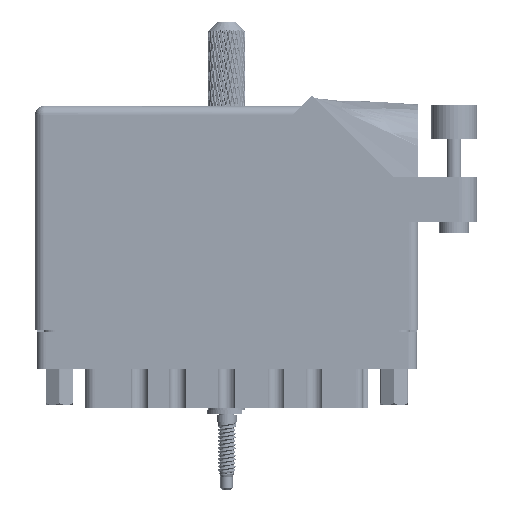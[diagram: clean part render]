
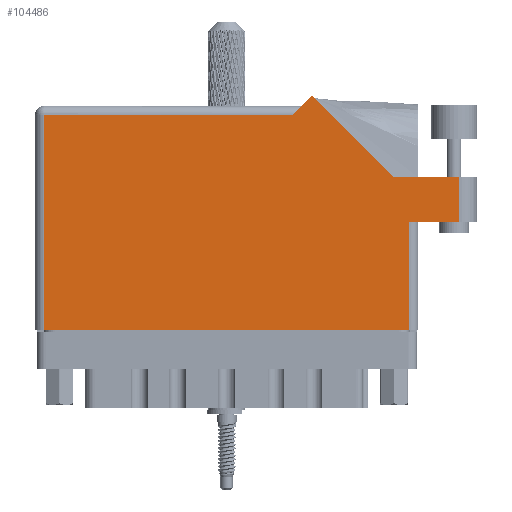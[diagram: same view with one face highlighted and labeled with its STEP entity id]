
A CAD part, front view. The second image highlights one B-rep face of the part: STEP entity #104486.
In plain terms, the highlighted face is planar.
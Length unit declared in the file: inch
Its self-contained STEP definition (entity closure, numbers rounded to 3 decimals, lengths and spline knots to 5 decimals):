
#1196 = LINE ( 'NONE', #117034, #110915 ) ;
#1963 = CARTESIAN_POINT ( 'NONE',  ( 2.55, 0., 0. ) ) ;
#3700 = VERTEX_POINT ( 'NONE', #48009 ) ;
#4929 = CARTESIAN_POINT ( 'NONE',  ( 3.012, 1.044, 0. ) ) ;
#5203 = EDGE_CURVE ( 'NONE', #57094, #62060, #86140, .T. ) ;
#5409 = EDGE_CURVE ( 'NONE', #79869, #85495, #1196, .T. ) ;
#7006 = ORIENTED_EDGE ( 'NONE', *, *, #32670, .T. ) ;
#7278 = DIRECTION ( 'NONE',  ( 0., 0., -1. ) ) ;
#7817 = VERTEX_POINT ( 'NONE', #110042 ) ;
#8028 = CARTESIAN_POINT ( 'NONE',  ( 0.062, 0., 0. ) ) ;
#8616 = VERTEX_POINT ( 'NONE', #47027 ) ;
#12531 = DIRECTION ( 'NONE',  ( -1., 0., 0. ) ) ;
#17126 = DIRECTION ( 'NONE',  ( 0., -1., 0. ) ) ;
#17730 = AXIS2_PLACEMENT_3D ( 'NONE', #115320, #7278, #95052 ) ;
#18593 = DIRECTION ( 'NONE',  ( 1., 0., 0. ) ) ;
#18639 = ORIENTED_EDGE ( 'NONE', *, *, #60508, .T. ) ;
#21123 = ORIENTED_EDGE ( 'NONE', *, *, #5409, .T. ) ;
#22456 = ORIENTED_EDGE ( 'NONE', *, *, #83307, .T. ) ;
#23489 = EDGE_CURVE ( 'NONE', #85495, #8616, #124495, .T. ) ;
#26390 = VECTOR ( 'NONE', #115205, 39.37008 ) ;
#27589 = CARTESIAN_POINT ( 'NONE',  ( 1.757, 1.468, 0. ) ) ;
#28414 = DIRECTION ( 'NONE',  ( -0.707, 0.707, 0. ) ) ;
#29213 = VERTEX_POINT ( 'NONE', #86836 ) ;
#31591 = VECTOR ( 'NONE', #28414, 39.37008 ) ;
#32055 = CARTESIAN_POINT ( 'NONE',  ( 2.887, 1.044, 0. ) ) ;
#32670 = EDGE_CURVE ( 'NONE', #8616, #7817, #53519, .T. ) ;
#35120 = ORIENTED_EDGE ( 'NONE', *, *, #47902, .T. ) ;
#39615 = DIRECTION ( 'NONE',  ( -0.707, -0.707, 0. ) ) ;
#47027 = CARTESIAN_POINT ( 'NONE',  ( 2.887, 0.737, 0. ) ) ;
#47902 = EDGE_CURVE ( 'NONE', #3700, #57094, #87890, .T. ) ;
#48009 = CARTESIAN_POINT ( 'NONE',  ( 1.88971, 1.60071, 0. ) ) ;
#48913 = CARTESIAN_POINT ( 'NONE',  ( 0., 1.468, 0. ) ) ;
#50754 = VECTOR ( 'NONE', #39615, 39.37008 ) ;
#50826 = ORIENTED_EDGE ( 'NONE', *, *, #23489, .T. ) ;
#53226 = EDGE_LOOP ( 'NONE', ( #50826, #7006, #22456, #83543, #35120, #107924, #18639, #68264, #21123 ) ) ;
#53519 = LINE ( 'NONE', #32055, #107724 ) ;
#57094 = VERTEX_POINT ( 'NONE', #27589 ) ;
#57649 = CARTESIAN_POINT ( 'NONE',  ( 2.44642, 1.044, 0. ) ) ;
#60508 = EDGE_CURVE ( 'NONE', #62060, #29213, #88337, .T. ) ;
#62060 = VERTEX_POINT ( 'NONE', #64249 ) ;
#62989 = DIRECTION ( 'NONE',  ( 0., 1., 0. ) ) ;
#64249 = CARTESIAN_POINT ( 'NONE',  ( 0.062, 1.468, 0. ) ) ;
#64496 = CARTESIAN_POINT ( 'NONE',  ( 2.55, 0.737, 0. ) ) ;
#68237 = CARTESIAN_POINT ( 'NONE',  ( 2.612, 0.737, 0. ) ) ;
#68264 = ORIENTED_EDGE ( 'NONE', *, *, #73088, .T. ) ;
#73088 = EDGE_CURVE ( 'NONE', #29213, #79869, #78944, .T. ) ;
#73712 = VECTOR ( 'NONE', #12531, 39.37008 ) ;
#78944 = LINE ( 'NONE', #107006, #26390 ) ;
#79869 = VERTEX_POINT ( 'NONE', #1963 ) ;
#83307 = EDGE_CURVE ( 'NONE', #7817, #120252, #83530, .T. ) ;
#83530 = LINE ( 'NONE', #4929, #126783 ) ;
#83543 = ORIENTED_EDGE ( 'NONE', *, *, #114080, .T. ) ;
#85495 = VERTEX_POINT ( 'NONE', #64496 ) ;
#86140 = LINE ( 'NONE', #48913, #73712 ) ;
#86810 = DIRECTION ( 'NONE',  ( 0., 1., 0. ) ) ;
#86836 = CARTESIAN_POINT ( 'NONE',  ( 0.062, 0., 0. ) ) ;
#87890 = LINE ( 'NONE', #88465, #50754 ) ;
#88337 = LINE ( 'NONE', #8028, #100730 ) ;
#88465 = CARTESIAN_POINT ( 'NONE',  ( 1.819, 1.53, 0. ) ) ;
#95052 = DIRECTION ( 'NONE',  ( -1., 0., 0. ) ) ;
#96975 = FACE_OUTER_BOUND ( 'NONE', #53226, .T. ) ;
#100730 = VECTOR ( 'NONE', #17126, 39.37008 ) ;
#103449 = DIRECTION ( 'NONE',  ( -1., 0., 0. ) ) ;
#104486 = ADVANCED_FACE ( 'NONE', ( #96975 ), #105840, .F. ) ;
#105840 = PLANE ( 'NONE',  #17730 ) ;
#107006 = CARTESIAN_POINT ( 'NONE',  ( 0., 0., 0. ) ) ;
#107320 = LINE ( 'NONE', #116981, #31591 ) ;
#107724 = VECTOR ( 'NONE', #62989, 39.37008 ) ;
#107924 = ORIENTED_EDGE ( 'NONE', *, *, #5203, .T. ) ;
#109015 = VECTOR ( 'NONE', #18593, 39.37008 ) ;
#110042 = CARTESIAN_POINT ( 'NONE',  ( 2.887, 1.044, 0. ) ) ;
#110915 = VECTOR ( 'NONE', #86810, 39.37008 ) ;
#114080 = EDGE_CURVE ( 'NONE', #120252, #3700, #107320, .T. ) ;
#115205 = DIRECTION ( 'NONE',  ( 1., 0., 0. ) ) ;
#115320 = CARTESIAN_POINT ( 'NONE',  ( 0., 1.53, 0. ) ) ;
#116981 = CARTESIAN_POINT ( 'NONE',  ( 2.44642, 1.044, 0. ) ) ;
#117034 = CARTESIAN_POINT ( 'NONE',  ( 2.55, 0.737, 0. ) ) ;
#120252 = VERTEX_POINT ( 'NONE', #57649 ) ;
#124495 = LINE ( 'NONE', #68237, #109015 ) ;
#126783 = VECTOR ( 'NONE', #103449, 39.37008 ) ;
